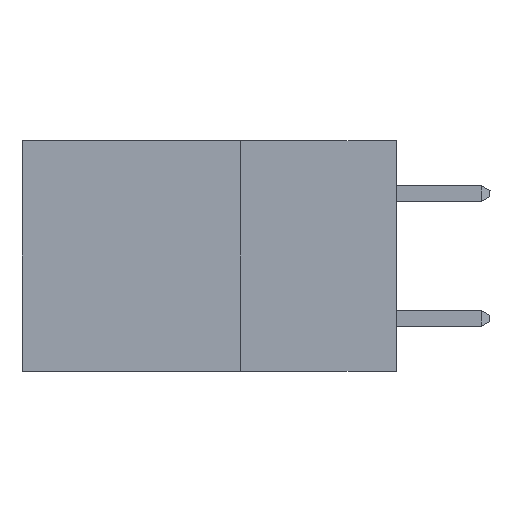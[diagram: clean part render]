
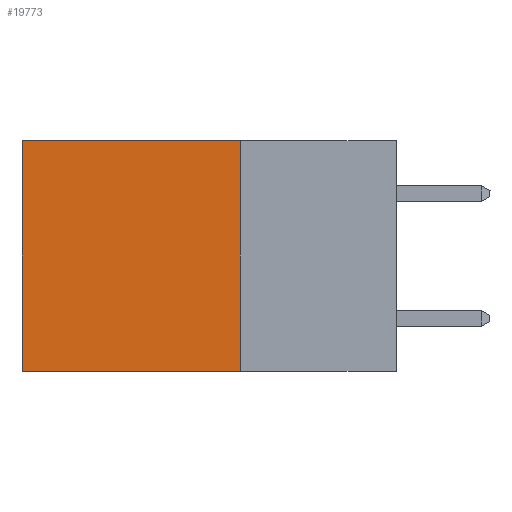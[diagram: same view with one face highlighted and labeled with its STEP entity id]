
A CAD part, left-side view. The second image highlights one B-rep face of the part: STEP entity #19773.
In plain terms, the highlighted planar face has unit normal (-1, 0, 0).
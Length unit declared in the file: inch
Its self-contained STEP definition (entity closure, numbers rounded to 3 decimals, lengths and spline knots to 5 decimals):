
#1301 = VECTOR ( 'NONE', #13596, 39.37008 ) ;
#1696 = CARTESIAN_POINT ( 'NONE',  ( 0.298, 0.25, 0. ) ) ;
#1773 = DIRECTION ( 'NONE',  ( 1., 0., 0. ) ) ;
#2022 = VERTEX_POINT ( 'NONE', #18729 ) ;
#4031 = VECTOR ( 'NONE', #15118, 39.37008 ) ;
#5025 = LINE ( 'NONE', #17071, #9170 ) ;
#5818 = ORIENTED_EDGE ( 'NONE', *, *, #9254, .T. ) ;
#5896 = EDGE_CURVE ( 'NONE', #22059, #19591, #5025, .T. ) ;
#6899 = LINE ( 'NONE', #22579, #20475 ) ;
#6913 = EDGE_CURVE ( 'NONE', #22059, #15660, #6899, .T. ) ;
#8138 = CARTESIAN_POINT ( 'NONE',  ( 0.298, 0.6, 0. ) ) ;
#9170 = VECTOR ( 'NONE', #22876, 39.37008 ) ;
#9254 = EDGE_CURVE ( 'NONE', #19591, #2022, #18151, .T. ) ;
#10708 = LINE ( 'NONE', #18992, #1301 ) ;
#11709 = ORIENTED_EDGE ( 'NONE', *, *, #6913, .F. ) ;
#11962 = CARTESIAN_POINT ( 'NONE',  ( 0.298, 0.25, 0. ) ) ;
#13029 = CARTESIAN_POINT ( 'NONE',  ( 0.298, 0.25, -0.37 ) ) ;
#13596 = DIRECTION ( 'NONE',  ( 0., 1., 0. ) ) ;
#14097 = DIRECTION ( 'NONE',  ( 0., 0., -1. ) ) ;
#15118 = DIRECTION ( 'NONE',  ( 0., 0., -1. ) ) ;
#15660 = VERTEX_POINT ( 'NONE', #13029 ) ;
#16374 = EDGE_LOOP ( 'NONE', ( #5818, #21670, #11709, #18132 ) ) ;
#17071 = CARTESIAN_POINT ( 'NONE',  ( 0.298, 0.25, 0. ) ) ;
#18132 = ORIENTED_EDGE ( 'NONE', *, *, #5896, .T. ) ;
#18151 = LINE ( 'NONE', #8138, #4031 ) ;
#18729 = CARTESIAN_POINT ( 'NONE',  ( 0.298, 0.6, -0.37 ) ) ;
#18972 = CARTESIAN_POINT ( 'NONE',  ( 0.298, 0.6, 0. ) ) ;
#18992 = CARTESIAN_POINT ( 'NONE',  ( 0.298, 0.25, -0.37 ) ) ;
#19517 = AXIS2_PLACEMENT_3D ( 'NONE', #1696, #1773, #14097 ) ;
#19558 = PLANE ( 'NONE',  #19517 ) ;
#19591 = VERTEX_POINT ( 'NONE', #18972 ) ;
#19773 = ADVANCED_FACE ( 'NONE', ( #20729 ), #19558, .F. ) ;
#20475 = VECTOR ( 'NONE', #22427, 39.37008 ) ;
#20729 = FACE_OUTER_BOUND ( 'NONE', #16374, .T. ) ;
#21330 = EDGE_CURVE ( 'NONE', #15660, #2022, #10708, .T. ) ;
#21670 = ORIENTED_EDGE ( 'NONE', *, *, #21330, .F. ) ;
#22059 = VERTEX_POINT ( 'NONE', #11962 ) ;
#22427 = DIRECTION ( 'NONE',  ( 0., 0., -1. ) ) ;
#22579 = CARTESIAN_POINT ( 'NONE',  ( 0.298, 0.25, 0. ) ) ;
#22876 = DIRECTION ( 'NONE',  ( 0., 1., 0. ) ) ;
